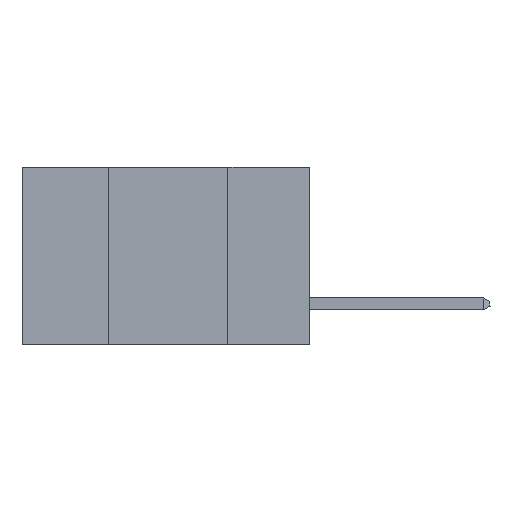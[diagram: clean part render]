
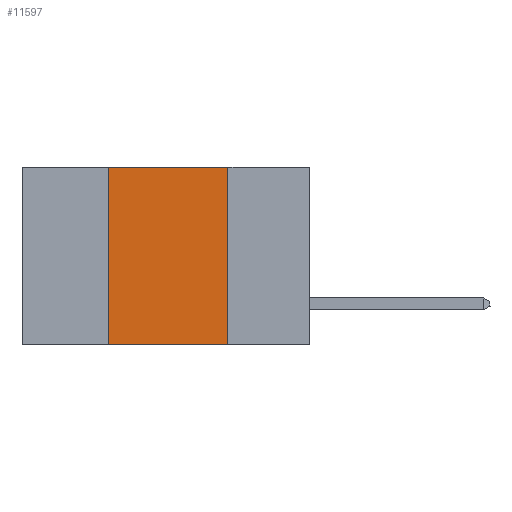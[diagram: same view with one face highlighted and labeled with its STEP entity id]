
A CAD part, left-side view. The second image highlights one B-rep face of the part: STEP entity #11597.
In plain terms, the highlighted planar face has unit normal (-1, 0, 0).
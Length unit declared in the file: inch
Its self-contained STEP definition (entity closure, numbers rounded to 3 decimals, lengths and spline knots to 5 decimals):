
#1860 = CARTESIAN_POINT ( 'NONE',  ( 0., 0.6, -0.37 ) ) ;
#2488 = PLANE ( 'NONE',  #8122 ) ;
#2568 = DIRECTION ( 'NONE',  ( 0., 0., 1. ) ) ;
#5456 = ORIENTED_EDGE ( 'NONE', *, *, #9622, .T. ) ;
#5817 = CARTESIAN_POINT ( 'NONE',  ( 0., 0.17, 0. ) ) ;
#6199 = EDGE_CURVE ( 'NONE', #23885, #14221, #15532, .T. ) ;
#7356 = ORIENTED_EDGE ( 'NONE', *, *, #11372, .F. ) ;
#7524 = LINE ( 'NONE', #1860, #22233 ) ;
#8122 = AXIS2_PLACEMENT_3D ( 'NONE', #24767, #10144, #11055 ) ;
#9622 = EDGE_CURVE ( 'NONE', #23885, #11014, #7524, .T. ) ;
#9737 = LINE ( 'NONE', #22160, #11189 ) ;
#10144 = DIRECTION ( 'NONE',  ( 1., 0., 0. ) ) ;
#10177 = ORIENTED_EDGE ( 'NONE', *, *, #24485, .F. ) ;
#11014 = VERTEX_POINT ( 'NONE', #15691 ) ;
#11055 = DIRECTION ( 'NONE',  ( 0., 0., -1. ) ) ;
#11189 = VECTOR ( 'NONE', #20222, 39.37008 ) ;
#11372 = EDGE_CURVE ( 'NONE', #26442, #11014, #9737, .T. ) ;
#11590 = DIRECTION ( 'NONE',  ( 0., -1., 0. ) ) ;
#11597 = ADVANCED_FACE ( 'NONE', ( #18421 ), #2488, .F. ) ;
#12137 = CARTESIAN_POINT ( 'NONE',  ( 0., 0.6, 0. ) ) ;
#12494 = CARTESIAN_POINT ( 'NONE',  ( 0., 0.42, -0.37 ) ) ;
#13018 = VECTOR ( 'NONE', #2568, 39.37008 ) ;
#14221 = VERTEX_POINT ( 'NONE', #23393 ) ;
#14426 = VECTOR ( 'NONE', #11590, 39.37008 ) ;
#15532 = LINE ( 'NONE', #23823, #13018 ) ;
#15691 = CARTESIAN_POINT ( 'NONE',  ( 0., 0.17, -0.37 ) ) ;
#17351 = EDGE_LOOP ( 'NONE', ( #7356, #10177, #26763, #5456 ) ) ;
#18421 = FACE_OUTER_BOUND ( 'NONE', #17351, .T. ) ;
#18475 = LINE ( 'NONE', #12137, #14426 ) ;
#20215 = DIRECTION ( 'NONE',  ( 0., -1., 0. ) ) ;
#20222 = DIRECTION ( 'NONE',  ( 0., 0., -1. ) ) ;
#22160 = CARTESIAN_POINT ( 'NONE',  ( 0., 0.17, 0. ) ) ;
#22233 = VECTOR ( 'NONE', #20215, 39.37008 ) ;
#23393 = CARTESIAN_POINT ( 'NONE',  ( 0., 0.42, 0. ) ) ;
#23823 = CARTESIAN_POINT ( 'NONE',  ( 0., 0.42, 0. ) ) ;
#23885 = VERTEX_POINT ( 'NONE', #12494 ) ;
#24485 = EDGE_CURVE ( 'NONE', #14221, #26442, #18475, .T. ) ;
#24767 = CARTESIAN_POINT ( 'NONE',  ( 0., 0.6, 0. ) ) ;
#26442 = VERTEX_POINT ( 'NONE', #5817 ) ;
#26763 = ORIENTED_EDGE ( 'NONE', *, *, #6199, .F. ) ;
